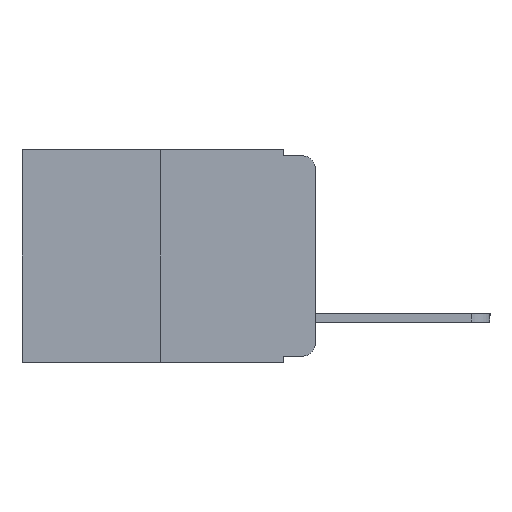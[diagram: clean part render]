
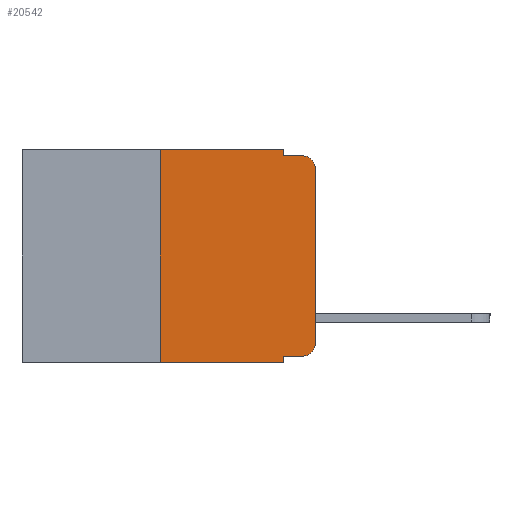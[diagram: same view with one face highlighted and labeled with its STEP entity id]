
A CAD part, left-side view. The second image highlights one B-rep face of the part: STEP entity #20542.
In plain terms, the highlighted planar face has unit normal (-1, 0, 0).
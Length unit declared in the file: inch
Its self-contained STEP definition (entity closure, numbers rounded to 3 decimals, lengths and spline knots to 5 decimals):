
#153 = CARTESIAN_POINT ( 'NONE',  ( 0., 0.25, -0.343 ) ) ;
#207 = EDGE_CURVE ( 'NONE', #18366, #10765, #7434, .T. ) ;
#525 = VERTEX_POINT ( 'NONE', #2343 ) ;
#1287 = CARTESIAN_POINT ( 'NONE',  ( 0., 0.051, -0.01 ) ) ;
#1463 = EDGE_CURVE ( 'NONE', #7236, #525, #10415, .T. ) ;
#1558 = VECTOR ( 'NONE', #20288, 39.37008 ) ;
#2312 = CARTESIAN_POINT ( 'NONE',  ( 0., 0.25, 0. ) ) ;
#2335 = DIRECTION ( 'NONE',  ( 0., 0., 1. ) ) ;
#2343 = CARTESIAN_POINT ( 'NONE',  ( 0., 0.25, 0. ) ) ;
#2640 = EDGE_CURVE ( 'NONE', #11101, #19777, #9612, .T. ) ;
#2995 = ORIENTED_EDGE ( 'NONE', *, *, #6056, .T. ) ;
#3126 = CARTESIAN_POINT ( 'NONE',  ( 0., 0.051, 0. ) ) ;
#3573 = DIRECTION ( 'NONE',  ( 0., -1., 0. ) ) ;
#3785 = EDGE_CURVE ( 'NONE', #19777, #17574, #20253, .T. ) ;
#3885 = VERTEX_POINT ( 'NONE', #10666 ) ;
#4924 = EDGE_CURVE ( 'NONE', #3885, #17574, #18221, .T. ) ;
#4934 = CARTESIAN_POINT ( 'NONE',  ( 0., 0.02, -0.313 ) ) ;
#5183 = ORIENTED_EDGE ( 'NONE', *, *, #1463, .F. ) ;
#5358 = VERTEX_POINT ( 'NONE', #6354 ) ;
#5749 = ORIENTED_EDGE ( 'NONE', *, *, #20728, .T. ) ;
#5872 = DIRECTION ( 'NONE',  ( 0., 0., 1. ) ) ;
#6056 = EDGE_CURVE ( 'NONE', #20678, #3885, #13034, .T. ) ;
#6066 = CARTESIAN_POINT ( 'NONE',  ( 0., 0.473, -0.343 ) ) ;
#6354 = CARTESIAN_POINT ( 'NONE',  ( 0., 0.02, -0.333 ) ) ;
#6638 = DIRECTION ( 'NONE',  ( 0., 0., -1. ) ) ;
#6738 = CARTESIAN_POINT ( 'NONE',  ( 0., 0.02, -0.03 ) ) ;
#6775 = AXIS2_PLACEMENT_3D ( 'NONE', #4934, #16547, #6638 ) ;
#6780 = ORIENTED_EDGE ( 'NONE', *, *, #207, .F. ) ;
#7236 = VERTEX_POINT ( 'NONE', #153 ) ;
#7434 = LINE ( 'NONE', #3126, #19980 ) ;
#7742 = ORIENTED_EDGE ( 'NONE', *, *, #4924, .T. ) ;
#8161 = LINE ( 'NONE', #6066, #20172 ) ;
#8408 = DIRECTION ( 'NONE',  ( 0., 0., -1. ) ) ;
#8446 = CARTESIAN_POINT ( 'NONE',  ( 0., 0.473, 0. ) ) ;
#8457 = CARTESIAN_POINT ( 'NONE',  ( 0., 0.473, 0. ) ) ;
#8638 = VECTOR ( 'NONE', #5872, 39.37008 ) ;
#9170 = CARTESIAN_POINT ( 'NONE',  ( 0., 0., 0. ) ) ;
#9612 = LINE ( 'NONE', #19599, #13985 ) ;
#9895 = VECTOR ( 'NONE', #2335, 39.37008 ) ;
#10085 = EDGE_CURVE ( 'NONE', #7236, #10765, #8161, .T. ) ;
#10096 = DIRECTION ( 'NONE',  ( 0., 0., -1. ) ) ;
#10104 = CARTESIAN_POINT ( 'NONE',  ( 0., 0.051, -0.343 ) ) ;
#10415 = LINE ( 'NONE', #2312, #9895 ) ;
#10516 = LINE ( 'NONE', #18703, #1558 ) ;
#10556 = AXIS2_PLACEMENT_3D ( 'NONE', #8446, #19882, #10096 ) ;
#10666 = CARTESIAN_POINT ( 'NONE',  ( 0., 0., -0.03 ) ) ;
#10765 = VERTEX_POINT ( 'NONE', #10104 ) ;
#10940 = DIRECTION ( 'NONE',  ( 0., -1., 0. ) ) ;
#11101 = VERTEX_POINT ( 'NONE', #20643 ) ;
#11113 = VECTOR ( 'NONE', #3573, 39.37008 ) ;
#11232 = ORIENTED_EDGE ( 'NONE', *, *, #18601, .T. ) ;
#12598 = EDGE_CURVE ( 'NONE', #525, #11101, #12920, .T. ) ;
#12920 = LINE ( 'NONE', #8457, #17315 ) ;
#13034 = LINE ( 'NONE', #9170, #8638 ) ;
#13348 = PLANE ( 'NONE',  #10556 ) ;
#13874 = EDGE_LOOP ( 'NONE', ( #2995, #7742, #18067, #20538, #16570, #5183, #18845, #6780, #5749, #11232 ) ) ;
#13985 = VECTOR ( 'NONE', #14798, 39.37008 ) ;
#14798 = DIRECTION ( 'NONE',  ( 0., 0., -1. ) ) ;
#15405 = DIRECTION ( 'NONE',  ( 0., 0., -1. ) ) ;
#15786 = CIRCLE ( 'NONE', #6775, 0.02 ) ;
#16547 = DIRECTION ( 'NONE',  ( -1., 0., 0. ) ) ;
#16570 = ORIENTED_EDGE ( 'NONE', *, *, #12598, .F. ) ;
#16877 = CARTESIAN_POINT ( 'NONE',  ( 0., 0.051, -0.01 ) ) ;
#17315 = VECTOR ( 'NONE', #19889, 39.37008 ) ;
#17503 = FACE_OUTER_BOUND ( 'NONE', #13874, .T. ) ;
#17574 = VERTEX_POINT ( 'NONE', #18332 ) ;
#18067 = ORIENTED_EDGE ( 'NONE', *, *, #3785, .F. ) ;
#18221 = CIRCLE ( 'NONE', #20083, 0.02 ) ;
#18261 = DIRECTION ( 'NONE',  ( -1., 0., 0. ) ) ;
#18332 = CARTESIAN_POINT ( 'NONE',  ( 0., 0.02, -0.01 ) ) ;
#18366 = VERTEX_POINT ( 'NONE', #18844 ) ;
#18601 = EDGE_CURVE ( 'NONE', #5358, #20678, #15786, .T. ) ;
#18629 = CARTESIAN_POINT ( 'NONE',  ( 0., 0., -0.313 ) ) ;
#18703 = CARTESIAN_POINT ( 'NONE',  ( 0., 0.051, -0.333 ) ) ;
#18844 = CARTESIAN_POINT ( 'NONE',  ( 0., 0.051, -0.333 ) ) ;
#18845 = ORIENTED_EDGE ( 'NONE', *, *, #10085, .T. ) ;
#19599 = CARTESIAN_POINT ( 'NONE',  ( 0., 0.051, 0. ) ) ;
#19777 = VERTEX_POINT ( 'NONE', #1287 ) ;
#19882 = DIRECTION ( 'NONE',  ( 1., 0., 0. ) ) ;
#19889 = DIRECTION ( 'NONE',  ( 0., -1., 0. ) ) ;
#19980 = VECTOR ( 'NONE', #15405, 39.37008 ) ;
#20083 = AXIS2_PLACEMENT_3D ( 'NONE', #6738, #18261, #8408 ) ;
#20172 = VECTOR ( 'NONE', #10940, 39.37008 ) ;
#20253 = LINE ( 'NONE', #16877, #11113 ) ;
#20288 = DIRECTION ( 'NONE',  ( 0., -1., 0. ) ) ;
#20538 = ORIENTED_EDGE ( 'NONE', *, *, #2640, .F. ) ;
#20542 = ADVANCED_FACE ( 'NONE', ( #17503 ), #13348, .F. ) ;
#20643 = CARTESIAN_POINT ( 'NONE',  ( 0., 0.051, 0. ) ) ;
#20678 = VERTEX_POINT ( 'NONE', #18629 ) ;
#20728 = EDGE_CURVE ( 'NONE', #18366, #5358, #10516, .T. ) ;
